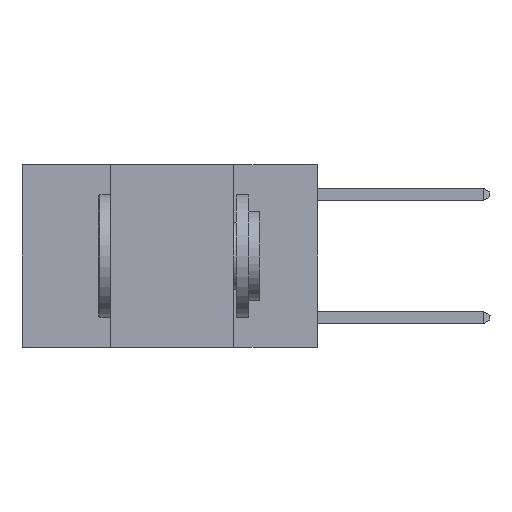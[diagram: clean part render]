
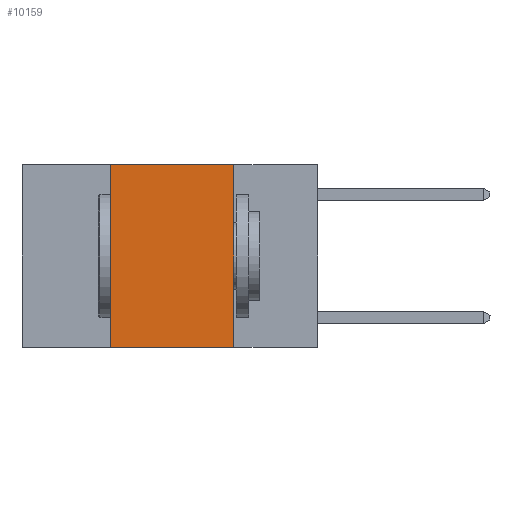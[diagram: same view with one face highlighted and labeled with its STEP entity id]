
A CAD part, left-side view. The second image highlights one B-rep face of the part: STEP entity #10159.
In plain terms, the highlighted planar face has unit normal (-1, 0, 0).
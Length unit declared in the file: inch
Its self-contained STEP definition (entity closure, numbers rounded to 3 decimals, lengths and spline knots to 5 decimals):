
#578 = ORIENTED_EDGE ( 'NONE', *, *, #13776, .T. ) ;
#1552 = DIRECTION ( 'NONE',  ( 0., -1., 0. ) ) ;
#2511 = EDGE_CURVE ( 'NONE', #15026, #2924, #10278, .T. ) ;
#2590 = CARTESIAN_POINT ( 'NONE',  ( 0., 0.6, -0.37 ) ) ;
#2924 = VERTEX_POINT ( 'NONE', #17036 ) ;
#3539 = VECTOR ( 'NONE', #1552, 39.37008 ) ;
#3649 = LINE ( 'NONE', #17140, #4521 ) ;
#3835 = ORIENTED_EDGE ( 'NONE', *, *, #2511, .F. ) ;
#3944 = DIRECTION ( 'NONE',  ( 0., -1., 0. ) ) ;
#4521 = VECTOR ( 'NONE', #9155, 39.37008 ) ;
#4847 = EDGE_CURVE ( 'NONE', #2924, #9156, #3649, .T. ) ;
#5216 = VECTOR ( 'NONE', #3944, 39.37008 ) ;
#5872 = EDGE_LOOP ( 'NONE', ( #14958, #3835, #10535, #578 ) ) ;
#6419 = DIRECTION ( 'NONE',  ( 0., 0., -1. ) ) ;
#6906 = CARTESIAN_POINT ( 'NONE',  ( 0., 0.42, 0. ) ) ;
#7141 = VECTOR ( 'NONE', #9568, 39.37008 ) ;
#8451 = CARTESIAN_POINT ( 'NONE',  ( 0., 0.17, -0.37 ) ) ;
#9155 = DIRECTION ( 'NONE',  ( 0., 0., -1. ) ) ;
#9156 = VERTEX_POINT ( 'NONE', #8451 ) ;
#9568 = DIRECTION ( 'NONE',  ( 0., 0., 1. ) ) ;
#9896 = VERTEX_POINT ( 'NONE', #14010 ) ;
#10159 = ADVANCED_FACE ( 'NONE', ( #16019 ), #13100, .F. ) ;
#10278 = LINE ( 'NONE', #10963, #3539 ) ;
#10535 = ORIENTED_EDGE ( 'NONE', *, *, #12517, .F. ) ;
#10963 = CARTESIAN_POINT ( 'NONE',  ( 0., 0.6, 0. ) ) ;
#11707 = AXIS2_PLACEMENT_3D ( 'NONE', #14404, #14465, #6419 ) ;
#12336 = LINE ( 'NONE', #2590, #5216 ) ;
#12517 = EDGE_CURVE ( 'NONE', #9896, #15026, #15185, .T. ) ;
#13100 = PLANE ( 'NONE',  #11707 ) ;
#13776 = EDGE_CURVE ( 'NONE', #9896, #9156, #12336, .T. ) ;
#14010 = CARTESIAN_POINT ( 'NONE',  ( 0., 0.42, -0.37 ) ) ;
#14138 = CARTESIAN_POINT ( 'NONE',  ( 0., 0.42, 0. ) ) ;
#14404 = CARTESIAN_POINT ( 'NONE',  ( 0., 0.6, 0. ) ) ;
#14465 = DIRECTION ( 'NONE',  ( 1., 0., 0. ) ) ;
#14958 = ORIENTED_EDGE ( 'NONE', *, *, #4847, .F. ) ;
#15026 = VERTEX_POINT ( 'NONE', #14138 ) ;
#15185 = LINE ( 'NONE', #6906, #7141 ) ;
#16019 = FACE_OUTER_BOUND ( 'NONE', #5872, .T. ) ;
#17036 = CARTESIAN_POINT ( 'NONE',  ( 0., 0.17, 0. ) ) ;
#17140 = CARTESIAN_POINT ( 'NONE',  ( 0., 0.17, 0. ) ) ;
